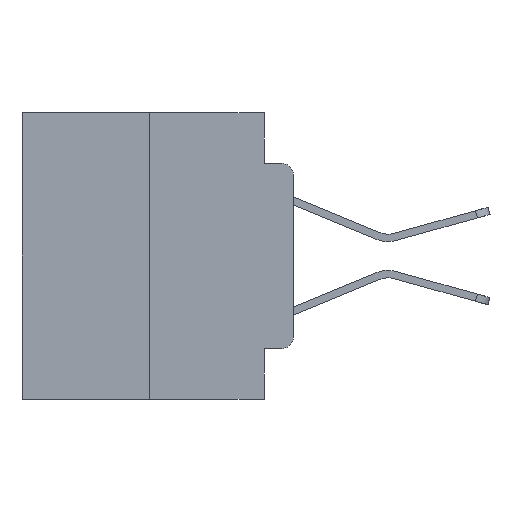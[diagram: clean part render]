
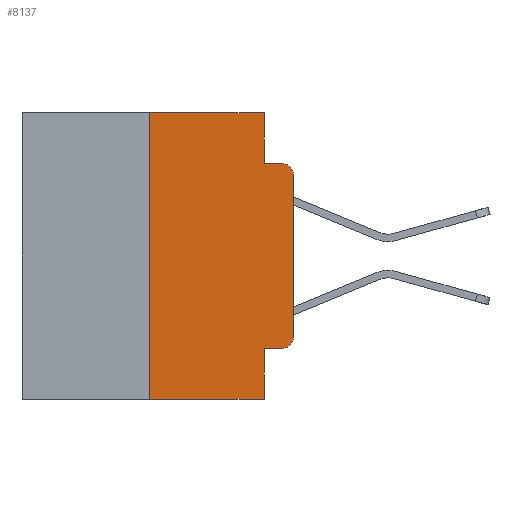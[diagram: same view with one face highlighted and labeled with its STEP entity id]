
A CAD part, left-side view. The second image highlights one B-rep face of the part: STEP entity #8137.
In plain terms, the highlighted planar face has unit normal (-1, 0, 0).
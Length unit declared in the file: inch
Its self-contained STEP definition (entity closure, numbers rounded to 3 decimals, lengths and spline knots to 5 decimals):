
#44 = VERTEX_POINT ( 'NONE', #9891 ) ;
#712 = CARTESIAN_POINT ( 'NONE',  ( 0., 0.473, 0. ) ) ;
#809 = CARTESIAN_POINT ( 'NONE',  ( 0., 0., -0.1085 ) ) ;
#1402 = AXIS2_PLACEMENT_3D ( 'NONE', #712, #7172, #22021 ) ;
#1739 = CARTESIAN_POINT ( 'NONE',  ( 0., 0.051, -0.0885 ) ) ;
#2048 = DIRECTION ( 'NONE',  ( 0., -1., 0. ) ) ;
#2199 = DIRECTION ( 'NONE',  ( 0., 0., -1. ) ) ;
#2322 = VERTEX_POINT ( 'NONE', #809 ) ;
#2520 = DIRECTION ( 'NONE',  ( -1., 0., 0. ) ) ;
#2832 = ORIENTED_EDGE ( 'NONE', *, *, #20357, .F. ) ;
#2872 = LINE ( 'NONE', #22077, #24780 ) ;
#3150 = VECTOR ( 'NONE', #2048, 39.37008 ) ;
#3483 = EDGE_CURVE ( 'NONE', #44, #2322, #21004, .T. ) ;
#3737 = CIRCLE ( 'NONE', #9702, 0.02 ) ;
#3790 = CARTESIAN_POINT ( 'NONE',  ( 0., 0.051, 0. ) ) ;
#3834 = CARTESIAN_POINT ( 'NONE',  ( 0., 0.02, -0.4115 ) ) ;
#3879 = DIRECTION ( 'NONE',  ( 0., -1., 0. ) ) ;
#3974 = EDGE_CURVE ( 'NONE', #12620, #27462, #20877, .T. ) ;
#4215 = CARTESIAN_POINT ( 'NONE',  ( 0., 0.25, -0.5 ) ) ;
#4305 = CARTESIAN_POINT ( 'NONE',  ( 0., 0.25, 0. ) ) ;
#4560 = VECTOR ( 'NONE', #6560, 39.37008 ) ;
#5031 = PLANE ( 'NONE',  #1402 ) ;
#6177 = CIRCLE ( 'NONE', #22924, 0.02 ) ;
#6518 = CARTESIAN_POINT ( 'NONE',  ( 0., 0.25, 0. ) ) ;
#6553 = DIRECTION ( 'NONE',  ( -1., 0., 0. ) ) ;
#6560 = DIRECTION ( 'NONE',  ( 0., 0., 1. ) ) ;
#6848 = ORIENTED_EDGE ( 'NONE', *, *, #15879, .T. ) ;
#7086 = VERTEX_POINT ( 'NONE', #13854 ) ;
#7172 = DIRECTION ( 'NONE',  ( 1., 0., 0. ) ) ;
#7664 = VERTEX_POINT ( 'NONE', #7766 ) ;
#7766 = CARTESIAN_POINT ( 'NONE',  ( 0., 0.051, -0.4115 ) ) ;
#8137 = ADVANCED_FACE ( 'NONE', ( #13419 ), #5031, .F. ) ;
#8147 = LINE ( 'NONE', #11807, #18781 ) ;
#8886 = VECTOR ( 'NONE', #2199, 39.37008 ) ;
#9129 = CARTESIAN_POINT ( 'NONE',  ( 0., 0.051, -0.5 ) ) ;
#9371 = DIRECTION ( 'NONE',  ( 0., -1., 0. ) ) ;
#9702 = AXIS2_PLACEMENT_3D ( 'NONE', #19293, #6553, #21417 ) ;
#9891 = CARTESIAN_POINT ( 'NONE',  ( 0., 0., -0.3915 ) ) ;
#11161 = CARTESIAN_POINT ( 'NONE',  ( 0., 0., 0. ) ) ;
#11252 = DIRECTION ( 'NONE',  ( 0., 0., 1. ) ) ;
#11807 = CARTESIAN_POINT ( 'NONE',  ( 0., 0.473, 0. ) ) ;
#12404 = DIRECTION ( 'NONE',  ( 0., 0., -1. ) ) ;
#12589 = VERTEX_POINT ( 'NONE', #27389 ) ;
#12620 = VERTEX_POINT ( 'NONE', #4215 ) ;
#13419 = FACE_OUTER_BOUND ( 'NONE', #22426, .T. ) ;
#13849 = ORIENTED_EDGE ( 'NONE', *, *, #21696, .F. ) ;
#13854 = CARTESIAN_POINT ( 'NONE',  ( 0., 0.051, -0.0885 ) ) ;
#13958 = DIRECTION ( 'NONE',  ( 0., -1., 0. ) ) ;
#14365 = VECTOR ( 'NONE', #12404, 39.37008 ) ;
#14511 = LINE ( 'NONE', #14830, #3150 ) ;
#14830 = CARTESIAN_POINT ( 'NONE',  ( 0., 0.051, -0.4115 ) ) ;
#15009 = CARTESIAN_POINT ( 'NONE',  ( 0., 0.051, 0. ) ) ;
#15335 = CARTESIAN_POINT ( 'NONE',  ( 0., 0.02, -0.3915 ) ) ;
#15408 = VECTOR ( 'NONE', #11252, 39.37008 ) ;
#15651 = VERTEX_POINT ( 'NONE', #3834 ) ;
#15850 = ORIENTED_EDGE ( 'NONE', *, *, #3974, .F. ) ;
#15879 = EDGE_CURVE ( 'NONE', #15651, #44, #6177, .T. ) ;
#16831 = ORIENTED_EDGE ( 'NONE', *, *, #16882, .F. ) ;
#16882 = EDGE_CURVE ( 'NONE', #20000, #7086, #19333, .T. ) ;
#17104 = ORIENTED_EDGE ( 'NONE', *, *, #18286, .F. ) ;
#17257 = VECTOR ( 'NONE', #3879, 39.37008 ) ;
#17434 = DIRECTION ( 'NONE',  ( 0., 0., -1. ) ) ;
#17955 = VERTEX_POINT ( 'NONE', #9129 ) ;
#18286 = EDGE_CURVE ( 'NONE', #7086, #12589, #22881, .T. ) ;
#18659 = EDGE_CURVE ( 'NONE', #12620, #17955, #2872, .T. ) ;
#18781 = VECTOR ( 'NONE', #13958, 39.37008 ) ;
#19293 = CARTESIAN_POINT ( 'NONE',  ( 0., 0.02, -0.1085 ) ) ;
#19333 = LINE ( 'NONE', #3790, #14365 ) ;
#20000 = VERTEX_POINT ( 'NONE', #26418 ) ;
#20357 = EDGE_CURVE ( 'NONE', #7664, #17955, #25772, .T. ) ;
#20877 = LINE ( 'NONE', #4305, #4560 ) ;
#21004 = LINE ( 'NONE', #11161, #15408 ) ;
#21140 = ORIENTED_EDGE ( 'NONE', *, *, #21239, .T. ) ;
#21239 = EDGE_CURVE ( 'NONE', #7664, #15651, #14511, .T. ) ;
#21417 = DIRECTION ( 'NONE',  ( 0., 0., -1. ) ) ;
#21696 = EDGE_CURVE ( 'NONE', #27462, #20000, #8147, .T. ) ;
#22021 = DIRECTION ( 'NONE',  ( 0., 0., -1. ) ) ;
#22077 = CARTESIAN_POINT ( 'NONE',  ( 0., 0.473, -0.5 ) ) ;
#22335 = ORIENTED_EDGE ( 'NONE', *, *, #3483, .T. ) ;
#22426 = EDGE_LOOP ( 'NONE', ( #22335, #22691, #17104, #16831, #13849, #15850, #23462, #2832, #21140, #6848 ) ) ;
#22542 = EDGE_CURVE ( 'NONE', #2322, #12589, #3737, .T. ) ;
#22691 = ORIENTED_EDGE ( 'NONE', *, *, #22542, .T. ) ;
#22881 = LINE ( 'NONE', #1739, #17257 ) ;
#22924 = AXIS2_PLACEMENT_3D ( 'NONE', #15335, #2520, #17434 ) ;
#23462 = ORIENTED_EDGE ( 'NONE', *, *, #18659, .T. ) ;
#24780 = VECTOR ( 'NONE', #9371, 39.37008 ) ;
#25772 = LINE ( 'NONE', #15009, #8886 ) ;
#26418 = CARTESIAN_POINT ( 'NONE',  ( 0., 0.051, 0. ) ) ;
#27389 = CARTESIAN_POINT ( 'NONE',  ( 0., 0.02, -0.0885 ) ) ;
#27462 = VERTEX_POINT ( 'NONE', #6518 ) ;
